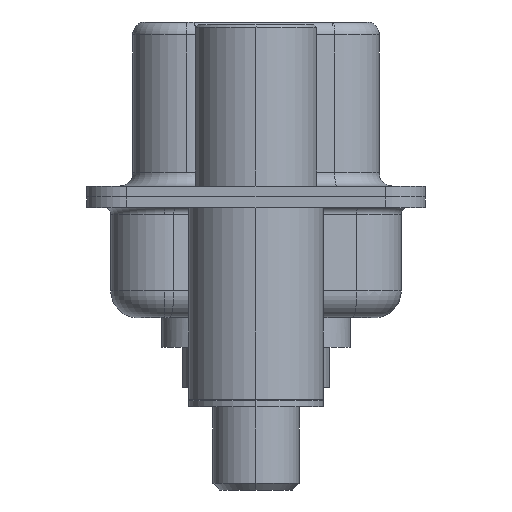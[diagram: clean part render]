
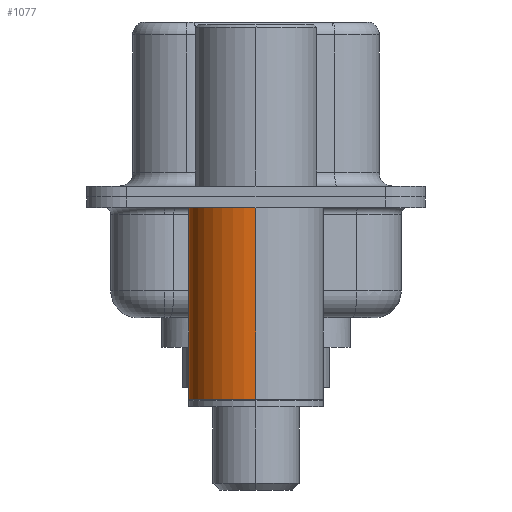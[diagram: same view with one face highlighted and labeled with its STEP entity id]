
A CAD part, left-side view. The second image highlights one B-rep face of the part: STEP entity #1077.
In plain terms, the highlighted cylindrical face has radius 2.5 mm (diameter 5 mm), a partial arc.
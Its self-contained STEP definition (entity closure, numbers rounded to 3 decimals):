
#134 = AXIS2_PLACEMENT_3D ( 'NONE', #412, #10073, #11466 ) ;
#288 = VECTOR ( 'NONE', #17602, 1000. ) ;
#412 = CARTESIAN_POINT ( 'NONE',  ( 0., 0., -7.525 ) ) ;
#477 = ORIENTED_EDGE ( 'NONE', *, *, #8255, .F. ) ;
#948 = DIRECTION ( 'NONE',  ( 1., 0., 0. ) ) ;
#1077 = ADVANCED_FACE ( 'NONE', ( #2532 ), #16798, .T. ) ;
#1675 = CARTESIAN_POINT ( 'NONE',  ( 0., 0., -0.4 ) ) ;
#2062 = LINE ( 'NONE', #10760, #288 ) ;
#2532 = FACE_OUTER_BOUND ( 'NONE', #11934, .T. ) ;
#3220 = EDGE_CURVE ( 'NONE', #14956, #6503, #14995, .T. ) ;
#4419 = CARTESIAN_POINT ( 'NONE',  ( 2.5, 0., -7.525 ) ) ;
#4646 = EDGE_CURVE ( 'NONE', #16317, #14956, #10089, .T. ) ;
#4717 = ORIENTED_EDGE ( 'NONE', *, *, #12085, .F. ) ;
#5226 = DIRECTION ( 'NONE',  ( 0., 0., 1. ) ) ;
#5270 = CIRCLE ( 'NONE', #7300, 2.5 ) ;
#5792 = DIRECTION ( 'NONE',  ( 0., 0., 1. ) ) ;
#6503 = VERTEX_POINT ( 'NONE', #6526 ) ;
#6526 = CARTESIAN_POINT ( 'NONE',  ( -2.5, 0., -0.4 ) ) ;
#7054 = DIRECTION ( 'NONE',  ( 1., 0., 0. ) ) ;
#7300 = AXIS2_PLACEMENT_3D ( 'NONE', #1675, #5792, #7054 ) ;
#7416 = CARTESIAN_POINT ( 'NONE',  ( -2.5, 0., -7.525 ) ) ;
#8255 = EDGE_CURVE ( 'NONE', #13220, #6503, #5270, .T. ) ;
#10073 = DIRECTION ( 'NONE',  ( 0., 0., 1. ) ) ;
#10089 = CIRCLE ( 'NONE', #134, 2.5 ) ;
#10147 = ORIENTED_EDGE ( 'NONE', *, *, #3220, .T. ) ;
#10652 = VECTOR ( 'NONE', #14793, 1000. ) ;
#10760 = CARTESIAN_POINT ( 'NONE',  ( 2.5, 0., 0.581 ) ) ;
#11466 = DIRECTION ( 'NONE',  ( 1., 0., 0. ) ) ;
#11843 = ORIENTED_EDGE ( 'NONE', *, *, #4646, .T. ) ;
#11934 = EDGE_LOOP ( 'NONE', ( #11843, #10147, #477, #4717 ) ) ;
#12085 = EDGE_CURVE ( 'NONE', #16317, #13220, #2062, .T. ) ;
#13220 = VERTEX_POINT ( 'NONE', #17778 ) ;
#13435 = CARTESIAN_POINT ( 'NONE',  ( -2.5, 0., 0.581 ) ) ;
#14331 = AXIS2_PLACEMENT_3D ( 'NONE', #16401, #5226, #948 ) ;
#14793 = DIRECTION ( 'NONE',  ( 0., 0., 1. ) ) ;
#14956 = VERTEX_POINT ( 'NONE', #7416 ) ;
#14995 = LINE ( 'NONE', #13435, #10652 ) ;
#16317 = VERTEX_POINT ( 'NONE', #4419 ) ;
#16401 = CARTESIAN_POINT ( 'NONE',  ( 0., 0., 0.581 ) ) ;
#16798 = CYLINDRICAL_SURFACE ( 'NONE', #14331, 2.5 ) ;
#17602 = DIRECTION ( 'NONE',  ( 0., 0., 1. ) ) ;
#17778 = CARTESIAN_POINT ( 'NONE',  ( 2.5, 0., -0.4 ) ) ;
